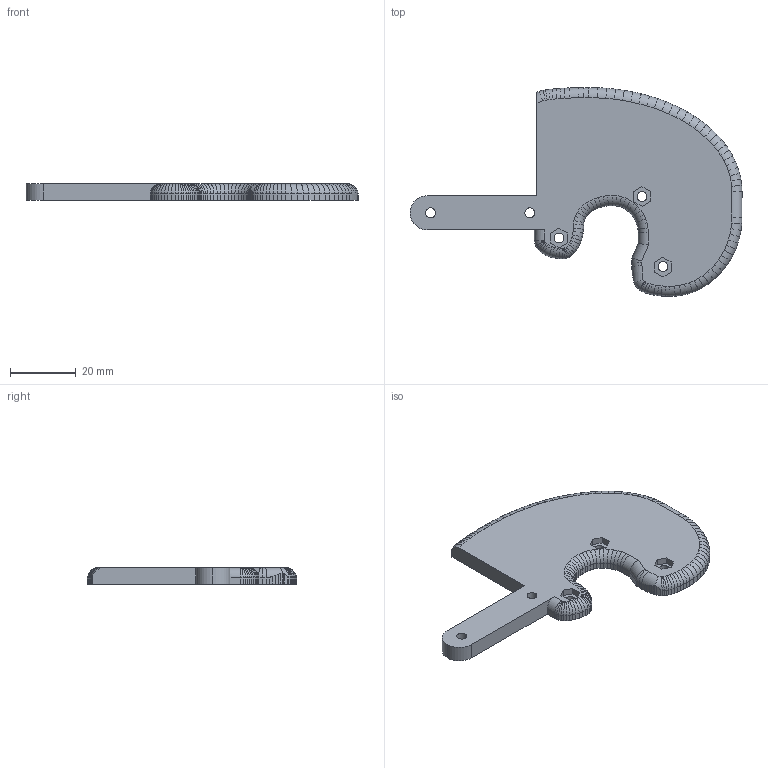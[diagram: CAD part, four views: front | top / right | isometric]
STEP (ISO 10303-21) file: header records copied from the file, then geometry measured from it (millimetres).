
FILE_DESCRIPTION (( 'STEP AP214' ), '1' );
FILE_NAME ('reprringerframeL.STEP', '2013-07-25T17:04:12', ( '' ), ( '' ), 'SwSTEP 2.0', 'SolidWorks 2013', '' );
FILE_SCHEMA (( 'AUTOMOTIVE_DESIGN' ));
Length unit declared in the file: inch
Products named in the file (1): reprringerframeL
Bounding box: 101.27 x 63.76 x 5 mm (x, y, z)
Volume: 15996.5 mm3; surface area: 8201.3 mm2
Topology: 1 solids, 1 shells, 300 faces, 762 edges, 467 vertices
Faces by surface type: plane 162, cylinder 138
Entity records: 15197 total; most frequent: CARTESIAN_POINT 4753, ORIENTED_EDGE 1524, DIRECTION 1095, EDGE_CURVE 762, VERTEX_POINT 467, LINE 443, VECTOR 443, AXIS2_PLACEMENT_3D 326
